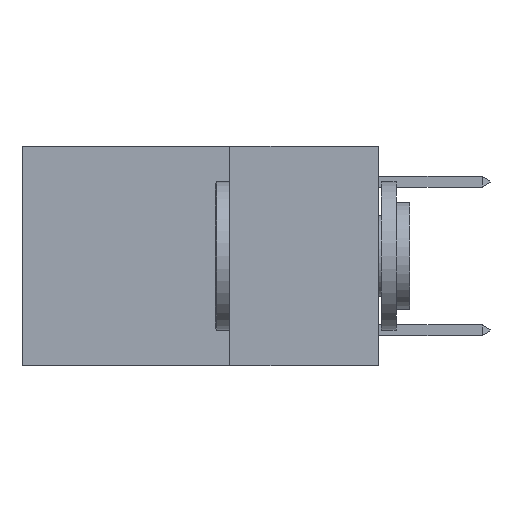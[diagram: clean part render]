
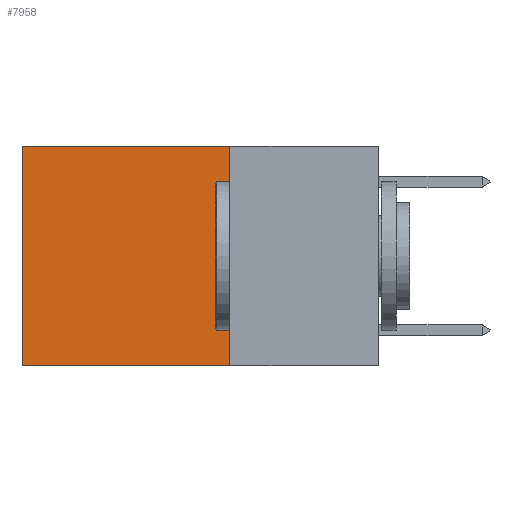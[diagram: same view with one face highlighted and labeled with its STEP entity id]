
A CAD part, left-side view. The second image highlights one B-rep face of the part: STEP entity #7958.
In plain terms, the highlighted planar face has unit normal (-1, 0, 0).
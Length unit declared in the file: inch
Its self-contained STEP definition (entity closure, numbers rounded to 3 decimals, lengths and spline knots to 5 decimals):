
#47 = DIRECTION ( 'NONE',  ( 0., 0., -1. ) ) ;
#266 = ORIENTED_EDGE ( 'NONE', *, *, #667, .T. ) ;
#667 = EDGE_CURVE ( 'NONE', #8528, #8150, #6121, .T. ) ;
#1564 = DIRECTION ( 'NONE',  ( 0., 0., -1. ) ) ;
#1896 = DIRECTION ( 'NONE',  ( 0., 1., 0. ) ) ;
#2132 = CARTESIAN_POINT ( 'NONE',  ( 0.2625, 0.6, -0.37 ) ) ;
#2154 = VECTOR ( 'NONE', #2856, 39.37008 ) ;
#2856 = DIRECTION ( 'NONE',  ( 0., 1., 0. ) ) ;
#4287 = CARTESIAN_POINT ( 'NONE',  ( 0.2625, 0.25, 0. ) ) ;
#4318 = CARTESIAN_POINT ( 'NONE',  ( 0.2625, 0.6, 0. ) ) ;
#5623 = EDGE_CURVE ( 'NONE', #8528, #6075, #9494, .T. ) ;
#5685 = VECTOR ( 'NONE', #8477, 39.37008 ) ;
#5726 = FACE_OUTER_BOUND ( 'NONE', #12466, .T. ) ;
#5865 = CARTESIAN_POINT ( 'NONE',  ( 0.2625, 0.25, 0. ) ) ;
#5905 = CARTESIAN_POINT ( 'NONE',  ( 0.2625, 0.25, -0.37 ) ) ;
#6075 = VERTEX_POINT ( 'NONE', #8760 ) ;
#6121 = LINE ( 'NONE', #12218, #2154 ) ;
#6234 = EDGE_CURVE ( 'NONE', #6075, #11866, #13454, .T. ) ;
#6764 = EDGE_CURVE ( 'NONE', #8150, #11866, #7574, .T. ) ;
#7053 = VECTOR ( 'NONE', #47, 39.37008 ) ;
#7254 = CARTESIAN_POINT ( 'NONE',  ( 0.2625, 0.6, 0. ) ) ;
#7574 = LINE ( 'NONE', #4318, #7053 ) ;
#7743 = ORIENTED_EDGE ( 'NONE', *, *, #6234, .F. ) ;
#7958 = ADVANCED_FACE ( 'NONE', ( #5726 ), #11007, .F. ) ;
#8150 = VERTEX_POINT ( 'NONE', #7254 ) ;
#8477 = DIRECTION ( 'NONE',  ( 0., 0., -1. ) ) ;
#8528 = VERTEX_POINT ( 'NONE', #11262 ) ;
#8760 = CARTESIAN_POINT ( 'NONE',  ( 0.2625, 0.25, -0.37 ) ) ;
#8993 = ORIENTED_EDGE ( 'NONE', *, *, #6764, .T. ) ;
#9494 = LINE ( 'NONE', #4287, #5685 ) ;
#10278 = VECTOR ( 'NONE', #1896, 39.37008 ) ;
#11007 = PLANE ( 'NONE',  #11199 ) ;
#11199 = AXIS2_PLACEMENT_3D ( 'NONE', #5865, #12112, #1564 ) ;
#11262 = CARTESIAN_POINT ( 'NONE',  ( 0.2625, 0.25, 0. ) ) ;
#11866 = VERTEX_POINT ( 'NONE', #2132 ) ;
#12112 = DIRECTION ( 'NONE',  ( 1., 0., 0. ) ) ;
#12218 = CARTESIAN_POINT ( 'NONE',  ( 0.2625, 0.25, 0. ) ) ;
#12329 = ORIENTED_EDGE ( 'NONE', *, *, #5623, .F. ) ;
#12466 = EDGE_LOOP ( 'NONE', ( #8993, #7743, #12329, #266 ) ) ;
#13454 = LINE ( 'NONE', #5905, #10278 ) ;
